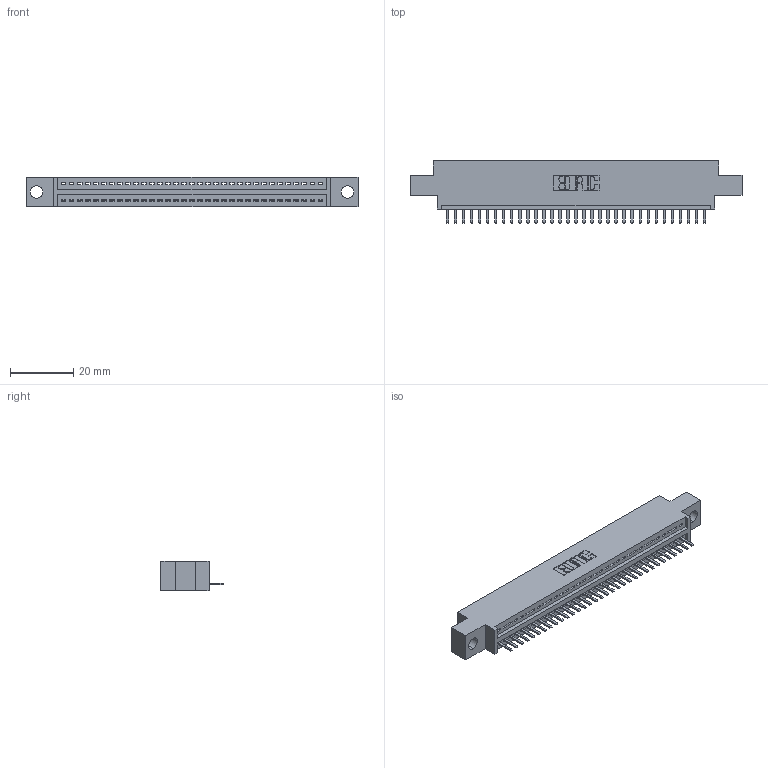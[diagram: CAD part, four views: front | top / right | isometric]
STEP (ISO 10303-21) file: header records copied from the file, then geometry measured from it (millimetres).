
FILE_DESCRIPTION (( 'STEP AP203' ), '1' );
FILE_NAME ('395-033-520-604.STEP', '2018-11-13T01:12:46', ( '' ), ( '' ), 'SwSTEP 2.0', 'SolidWorks 2016', '' );
FILE_SCHEMA (( 'CONFIG_CONTROL_DESIGN' ));
Length unit declared in the file: inch
Products named in the file (3): 395-033-520-604; 345 Part_0.170 Offset - 0.156 Dia-TH; 345-292-001_345-293-120
Assembly tree (34 placements, depth 2):
  395-033-520-604
    345 Part_0.170 Offset - 0.156 Dia-TH
    345-292-001_345-293-120  x33
Bounding box: 105.03 x 19.68 x 9.4 mm (x, y, z)
Volume: 9605.9 mm3; surface area: 12267.8 mm2
Topology: 34 solids, 34 shells, 2176 faces, 6425 edges, 4194 vertices
Faces by surface type: plane 1470, cylinder 706
Entity records: 26297 total; most frequent: CARTESIAN_POINT 4575, ORIENTED_EDGE 4530, DIRECTION 3995, EDGE_CURVE 2265, VECTOR 1997, LINE 1997, VERTEX_POINT 1506, AXIS2_PLACEMENT_3D 999
